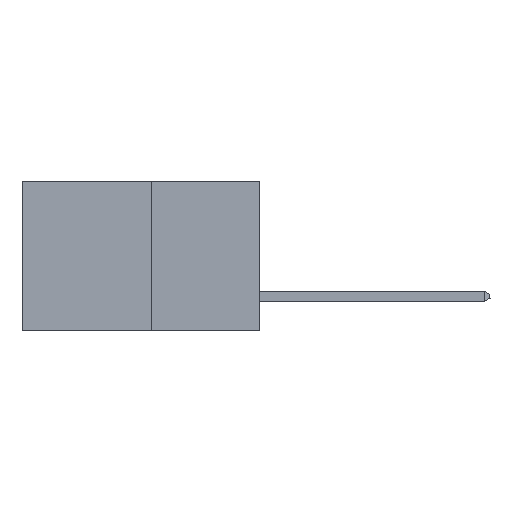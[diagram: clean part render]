
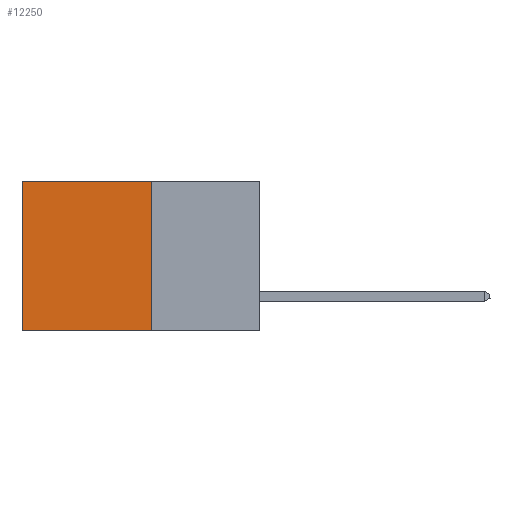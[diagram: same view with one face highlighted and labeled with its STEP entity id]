
A CAD part, left-side view. The second image highlights one B-rep face of the part: STEP entity #12250.
In plain terms, the highlighted planar face has unit normal (-1, 0, 0).
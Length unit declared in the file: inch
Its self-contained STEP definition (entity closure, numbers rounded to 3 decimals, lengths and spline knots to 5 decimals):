
#1401 = VECTOR ( 'NONE', #5760, 39.37008 ) ;
#2797 = CARTESIAN_POINT ( 'NONE',  ( 0.277, 0.27, -0.37 ) ) ;
#4018 = ORIENTED_EDGE ( 'NONE', *, *, #13985, .T. ) ;
#4759 = DIRECTION ( 'NONE',  ( 0., 0., -1. ) ) ;
#5314 = EDGE_CURVE ( 'NONE', #10954, #12593, #17814, .T. ) ;
#5390 = VECTOR ( 'NONE', #4759, 39.37008 ) ;
#5760 = DIRECTION ( 'NONE',  ( 0., 1., 0. ) ) ;
#7362 = DIRECTION ( 'NONE',  ( 0., 1., 0. ) ) ;
#7474 = LINE ( 'NONE', #19497, #15163 ) ;
#8205 = ORIENTED_EDGE ( 'NONE', *, *, #5314, .F. ) ;
#8352 = CARTESIAN_POINT ( 'NONE',  ( 0.277, 0.59, -0.37 ) ) ;
#9109 = PLANE ( 'NONE',  #12649 ) ;
#9425 = CARTESIAN_POINT ( 'NONE',  ( 0.277, 0.59, -0.37 ) ) ;
#9577 = LINE ( 'NONE', #9425, #5390 ) ;
#10046 = CARTESIAN_POINT ( 'NONE',  ( 0.277, 0.27, -0.37 ) ) ;
#10515 = VERTEX_POINT ( 'NONE', #10616 ) ;
#10616 = CARTESIAN_POINT ( 'NONE',  ( 0.277, 0.27, 0. ) ) ;
#10695 = DIRECTION ( 'NONE',  ( 0., 0., -1. ) ) ;
#10954 = VERTEX_POINT ( 'NONE', #10046 ) ;
#11130 = EDGE_CURVE ( 'NONE', #10515, #10954, #7474, .T. ) ;
#11343 = VECTOR ( 'NONE', #7362, 39.37008 ) ;
#11489 = ORIENTED_EDGE ( 'NONE', *, *, #12846, .T. ) ;
#11630 = EDGE_LOOP ( 'NONE', ( #4018, #8205, #19859, #11489 ) ) ;
#11990 = DIRECTION ( 'NONE',  ( 0., 0., -1. ) ) ;
#12250 = ADVANCED_FACE ( 'NONE', ( #14408 ), #9109, .F. ) ;
#12593 = VERTEX_POINT ( 'NONE', #8352 ) ;
#12649 = AXIS2_PLACEMENT_3D ( 'NONE', #2797, #19714, #10695 ) ;
#12846 = EDGE_CURVE ( 'NONE', #10515, #14224, #19368, .T. ) ;
#13985 = EDGE_CURVE ( 'NONE', #14224, #12593, #9577, .T. ) ;
#14224 = VERTEX_POINT ( 'NONE', #19033 ) ;
#14408 = FACE_OUTER_BOUND ( 'NONE', #11630, .T. ) ;
#15027 = CARTESIAN_POINT ( 'NONE',  ( 0.277, 0.27, 0. ) ) ;
#15163 = VECTOR ( 'NONE', #11990, 39.37008 ) ;
#17814 = LINE ( 'NONE', #18032, #1401 ) ;
#18032 = CARTESIAN_POINT ( 'NONE',  ( 0.277, 0.27, -0.37 ) ) ;
#19033 = CARTESIAN_POINT ( 'NONE',  ( 0.277, 0.59, 0. ) ) ;
#19368 = LINE ( 'NONE', #15027, #11343 ) ;
#19497 = CARTESIAN_POINT ( 'NONE',  ( 0.277, 0.27, -0.37 ) ) ;
#19714 = DIRECTION ( 'NONE',  ( 1., 0., 0. ) ) ;
#19859 = ORIENTED_EDGE ( 'NONE', *, *, #11130, .F. ) ;
